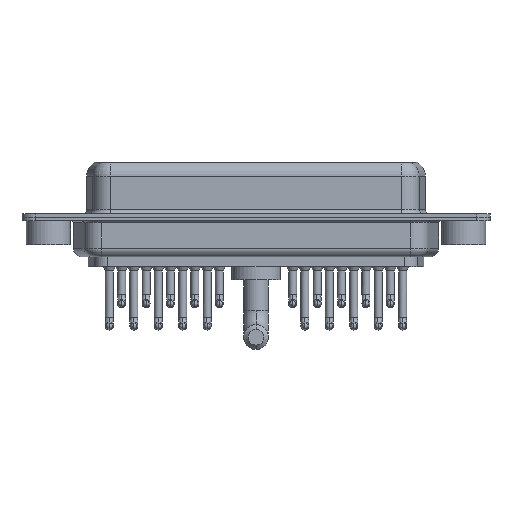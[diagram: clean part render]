
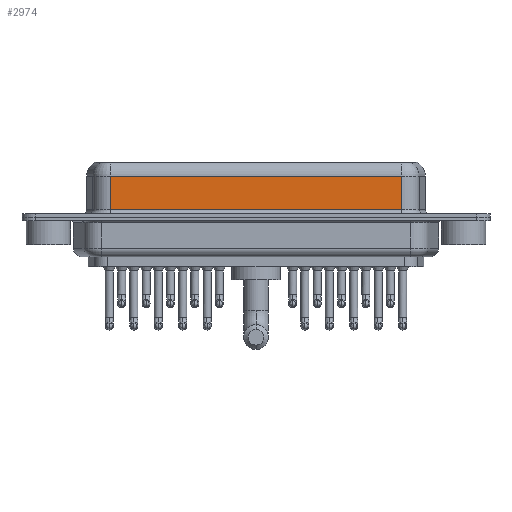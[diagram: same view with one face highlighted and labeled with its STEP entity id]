
A CAD part, front view. The second image highlights one B-rep face of the part: STEP entity #2974.
In plain terms, the highlighted planar face has unit normal (0, -1, 0).
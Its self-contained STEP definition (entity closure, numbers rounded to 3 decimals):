
#23 = VECTOR ( 'NONE', #1074, 1000. ) ;
#921 = VERTEX_POINT ( 'NONE', #8229 ) ;
#1074 = DIRECTION ( 'NONE',  ( 1., 0., 0. ) ) ;
#2226 = DIRECTION ( 'NONE',  ( -1., 0., 0. ) ) ;
#2449 = LINE ( 'NONE', #7829, #19767 ) ;
#2939 = VERTEX_POINT ( 'NONE', #12081 ) ;
#2974 = ADVANCED_FACE ( 'NONE', ( #6803 ), #22266, .F. ) ;
#3302 = VERTEX_POINT ( 'NONE', #18479 ) ;
#4396 = EDGE_CURVE ( 'NONE', #921, #2939, #17910, .T. ) ;
#4976 = CARTESIAN_POINT ( 'NONE',  ( 40.037, -3.95, 6.4 ) ) ;
#5854 = DIRECTION ( 'NONE',  ( 0., 0., -1. ) ) ;
#6790 = ORIENTED_EDGE ( 'NONE', *, *, #15141, .F. ) ;
#6803 = FACE_OUTER_BOUND ( 'NONE', #7561, .T. ) ;
#7133 = LINE ( 'NONE', #7716, #23 ) ;
#7561 = EDGE_LOOP ( 'NONE', ( #6790, #15875, #22528, #21584 ) ) ;
#7716 = CARTESIAN_POINT ( 'NONE',  ( 40.037, -3.95, 0.9 ) ) ;
#7829 = CARTESIAN_POINT ( 'NONE',  ( 7.013, -3.95, 6.4 ) ) ;
#7910 = CARTESIAN_POINT ( 'NONE',  ( 40.037, -3.95, 6.4 ) ) ;
#8229 = CARTESIAN_POINT ( 'NONE',  ( 40.037, -3.95, 4.65 ) ) ;
#8328 = VECTOR ( 'NONE', #2226, 1000. ) ;
#9535 = DIRECTION ( 'NONE',  ( 0., 0., -1. ) ) ;
#12081 = CARTESIAN_POINT ( 'NONE',  ( 7.013, -3.95, 4.65 ) ) ;
#12882 = CARTESIAN_POINT ( 'NONE',  ( 40.037, -3.95, 4.65 ) ) ;
#13344 = DIRECTION ( 'NONE',  ( 0., 0., 1. ) ) ;
#13452 = DIRECTION ( 'NONE',  ( 0., 1., 0. ) ) ;
#14111 = AXIS2_PLACEMENT_3D ( 'NONE', #4976, #13452, #13344 ) ;
#14595 = EDGE_CURVE ( 'NONE', #3302, #20242, #7133, .T. ) ;
#14764 = EDGE_CURVE ( 'NONE', #2939, #3302, #2449, .T. ) ;
#15141 = EDGE_CURVE ( 'NONE', #921, #20242, #21656, .T. ) ;
#15875 = ORIENTED_EDGE ( 'NONE', *, *, #4396, .T. ) ;
#16711 = CARTESIAN_POINT ( 'NONE',  ( 40.037, -3.95, 0.9 ) ) ;
#17910 = LINE ( 'NONE', #12882, #8328 ) ;
#18479 = CARTESIAN_POINT ( 'NONE',  ( 7.013, -3.95, 0.9 ) ) ;
#19767 = VECTOR ( 'NONE', #9535, 1000. ) ;
#20242 = VERTEX_POINT ( 'NONE', #16711 ) ;
#21238 = VECTOR ( 'NONE', #5854, 1000. ) ;
#21584 = ORIENTED_EDGE ( 'NONE', *, *, #14595, .T. ) ;
#21656 = LINE ( 'NONE', #7910, #21238 ) ;
#22266 = PLANE ( 'NONE',  #14111 ) ;
#22528 = ORIENTED_EDGE ( 'NONE', *, *, #14764, .T. ) ;
